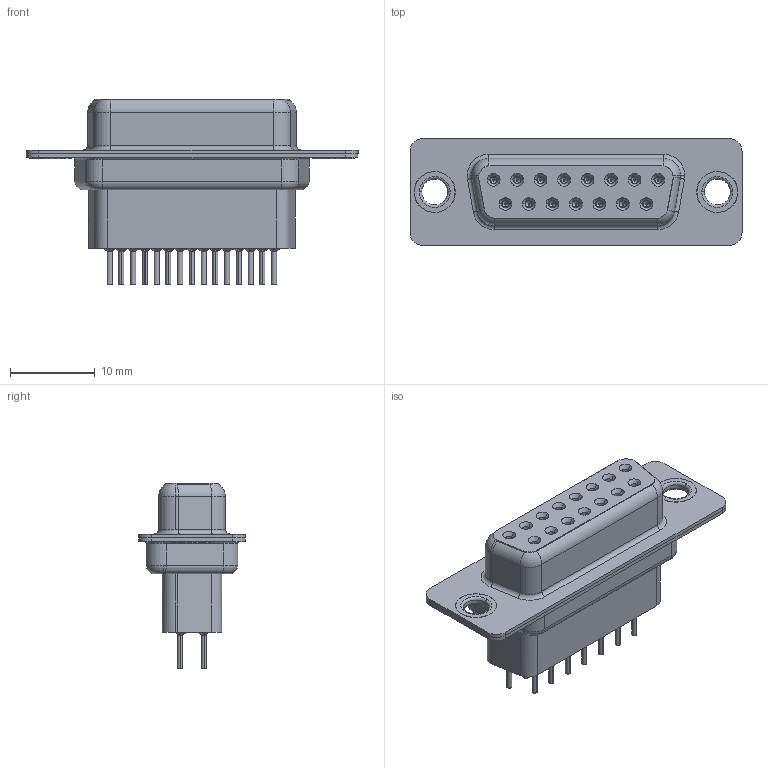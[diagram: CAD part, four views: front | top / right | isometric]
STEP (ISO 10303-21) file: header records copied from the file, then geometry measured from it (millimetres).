
FILE_DESCRIPTION (( 'STEP AP203' ), '1' );
FILE_NAME ('628-015-221-051.STEP', '2020-07-13T23:30:26', ( '' ), ( '' ), 'SwSTEP 2.0', 'SolidWorks 2020', '' );
FILE_SCHEMA (( 'CONFIG_CONTROL_DESIGN' ));
Length unit declared in the file: millimetre
Products named in the file (7): 628 Contact Row 2_21H; 628-015-221-051; 628 Shell Rear_15 Contacts; 628 Thru Hole Rivet; 628 Housing_15 HP; 628 Shell Front_15 Contacts; 628 Contact Row 1_21H
Assembly tree (20 placements, depth 2):
  628-015-221-051
    628 Housing_15 HP
    628 Shell Front_15 Contacts
    628 Shell Rear_15 Contacts
    628 Contact Row 1_21H  x8
    628 Contact Row 2_21H  x7
    628 Thru Hole Rivet  x2
Bounding box: 39.15 x 12.6 x 21.9 mm (x, y, z)
Volume: 3195.1 mm3; surface area: 7500.6 mm2
Topology: 20 solids, 20 shells, 2098 faces, 5343 edges, 3326 vertices
Faces by surface type: cylinder 616, plane 532, torus 425, bspline 300, cone 225
Entity records: 22115 total; most frequent: CARTESIAN_POINT 5755, DIRECTION 3341, ORIENTED_EDGE 3114, EDGE_CURVE 1557, AXIS2_PLACEMENT_3D 1392, VERTEX_POINT 975, CIRCLE 761, EDGE_LOOP 746
